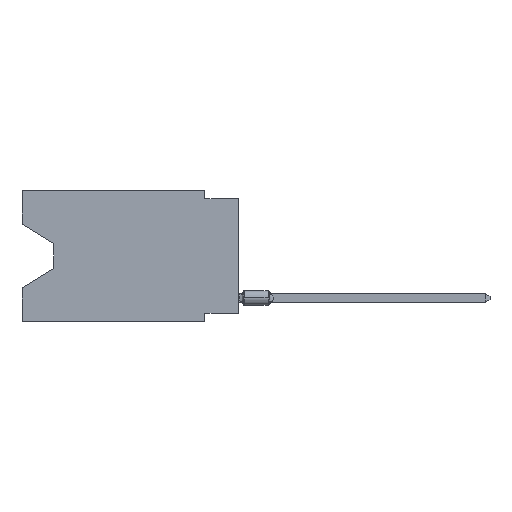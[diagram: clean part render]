
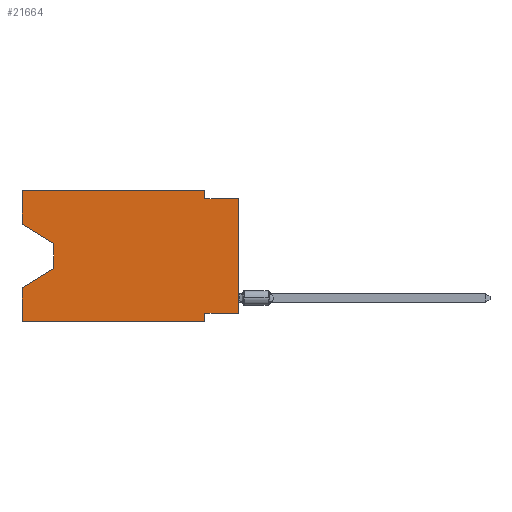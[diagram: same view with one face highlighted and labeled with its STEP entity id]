
A CAD part, left-side view. The second image highlights one B-rep face of the part: STEP entity #21664.
In plain terms, the highlighted planar face has unit normal (-1, 0, 0).
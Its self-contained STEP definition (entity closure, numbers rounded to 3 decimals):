
#264 = CARTESIAN_POINT ( 'NONE',  ( 0., 2.54, -0.635 ) ) ;
#439 = CARTESIAN_POINT ( 'NONE',  ( 0., 16.383, -2.546 ) ) ;
#1174 = VECTOR ( 'NONE', #18833, 1000. ) ;
#1178 = EDGE_CURVE ( 'NONE', #4654, #1676, #14690, .T. ) ;
#1676 = VERTEX_POINT ( 'NONE', #264 ) ;
#3243 = EDGE_CURVE ( 'NONE', #1676, #13821, #23773, .T. ) ;
#3281 = VECTOR ( 'NONE', #22348, 1000. ) ;
#4212 = VECTOR ( 'NONE', #21078, 1000. ) ;
#4266 = ORIENTED_EDGE ( 'NONE', *, *, #9920, .F. ) ;
#4325 = EDGE_CURVE ( 'NONE', #22542, #16185, #16788, .T. ) ;
#4528 = ORIENTED_EDGE ( 'NONE', *, *, #1178, .F. ) ;
#4582 = EDGE_CURVE ( 'NONE', #15624, #26573, #26738, .T. ) ;
#4654 = VERTEX_POINT ( 'NONE', #21216 ) ;
#4695 = DIRECTION ( 'NONE',  ( 0., -1., 0. ) ) ;
#4737 = EDGE_CURVE ( 'NONE', #22542, #13821, #25734, .T. ) ;
#5207 = EDGE_CURVE ( 'NONE', #12512, #17595, #5778, .T. ) ;
#5304 = DIRECTION ( 'NONE',  ( 0., 0., -1. ) ) ;
#5778 = LINE ( 'NONE', #7479, #24340 ) ;
#6340 = EDGE_CURVE ( 'NONE', #16185, #13503, #12993, .T. ) ;
#6423 = CARTESIAN_POINT ( 'NONE',  ( 0., 0., 0. ) ) ;
#6930 = VECTOR ( 'NONE', #19322, 1000. ) ;
#7479 = CARTESIAN_POINT ( 'NONE',  ( 0., 16.383, 0. ) ) ;
#7759 = CARTESIAN_POINT ( 'NONE',  ( 0., 16.383, 0. ) ) ;
#8341 = DIRECTION ( 'NONE',  ( 0., 0., -1. ) ) ;
#8631 = CARTESIAN_POINT ( 'NONE',  ( 0., 2.54, -9.906 ) ) ;
#8984 = VERTEX_POINT ( 'NONE', #7759 ) ;
#9226 = VECTOR ( 'NONE', #19690, 1000. ) ;
#9525 = CARTESIAN_POINT ( 'NONE',  ( 0., 16.383, -2.546 ) ) ;
#9920 = EDGE_CURVE ( 'NONE', #12831, #8984, #21634, .T. ) ;
#10760 = EDGE_CURVE ( 'NONE', #12831, #15624, #23974, .T. ) ;
#10925 = VECTOR ( 'NONE', #25218, 1000. ) ;
#10999 = CARTESIAN_POINT ( 'NONE',  ( 0., 2.54, -9.271 ) ) ;
#11297 = CARTESIAN_POINT ( 'NONE',  ( 0., 2.54, -9.906 ) ) ;
#11375 = CARTESIAN_POINT ( 'NONE',  ( 0., 0., -0.635 ) ) ;
#11657 = FACE_OUTER_BOUND ( 'NONE', #24232, .T. ) ;
#12475 = ORIENTED_EDGE ( 'NONE', *, *, #22771, .T. ) ;
#12502 = LINE ( 'NONE', #21076, #1174 ) ;
#12512 = VERTEX_POINT ( 'NONE', #18437 ) ;
#12831 = VERTEX_POINT ( 'NONE', #9525 ) ;
#12993 = LINE ( 'NONE', #8631, #6930 ) ;
#13197 = CARTESIAN_POINT ( 'NONE',  ( 0., 16.383, -7.36 ) ) ;
#13226 = LINE ( 'NONE', #15622, #9226 ) ;
#13503 = VERTEX_POINT ( 'NONE', #11297 ) ;
#13821 = VERTEX_POINT ( 'NONE', #19160 ) ;
#14046 = CARTESIAN_POINT ( 'NONE',  ( 0., 13.97, -4.013 ) ) ;
#14049 = DIRECTION ( 'NONE',  ( 1., 0., 0. ) ) ;
#14084 = AXIS2_PLACEMENT_3D ( 'NONE', #22908, #14049, #5304 ) ;
#14263 = ORIENTED_EDGE ( 'NONE', *, *, #10760, .T. ) ;
#14690 = LINE ( 'NONE', #19448, #17279 ) ;
#15227 = CARTESIAN_POINT ( 'NONE',  ( 0., 13.97, -5.893 ) ) ;
#15622 = CARTESIAN_POINT ( 'NONE',  ( 0., 16.383, -9.906 ) ) ;
#15624 = VERTEX_POINT ( 'NONE', #17982 ) ;
#15697 = CARTESIAN_POINT ( 'NONE',  ( 0., 16.383, 0. ) ) ;
#16185 = VERTEX_POINT ( 'NONE', #10999 ) ;
#16788 = LINE ( 'NONE', #21005, #23091 ) ;
#17279 = VECTOR ( 'NONE', #8341, 1000. ) ;
#17595 = VERTEX_POINT ( 'NONE', #13197 ) ;
#17880 = ORIENTED_EDGE ( 'NONE', *, *, #4325, .F. ) ;
#17982 = CARTESIAN_POINT ( 'NONE',  ( 0., 13.97, -4.013 ) ) ;
#18437 = CARTESIAN_POINT ( 'NONE',  ( 0., 16.383, -9.906 ) ) ;
#18833 = DIRECTION ( 'NONE',  ( 0., 0.855, -0.519 ) ) ;
#18965 = ORIENTED_EDGE ( 'NONE', *, *, #4582, .T. ) ;
#19160 = CARTESIAN_POINT ( 'NONE',  ( 0., 0., -0.635 ) ) ;
#19322 = DIRECTION ( 'NONE',  ( 0., 0., -1. ) ) ;
#19387 = ORIENTED_EDGE ( 'NONE', *, *, #4737, .T. ) ;
#19448 = CARTESIAN_POINT ( 'NONE',  ( 0., 2.54, 0. ) ) ;
#19564 = ORIENTED_EDGE ( 'NONE', *, *, #23654, .F. ) ;
#19690 = DIRECTION ( 'NONE',  ( 0., -1., 0. ) ) ;
#19952 = DIRECTION ( 'NONE',  ( 0., -1., 0. ) ) ;
#20038 = LINE ( 'NONE', #15697, #27733 ) ;
#20232 = PLANE ( 'NONE',  #14084 ) ;
#20842 = CARTESIAN_POINT ( 'NONE',  ( 0., 16.383, 0. ) ) ;
#20847 = DIRECTION ( 'NONE',  ( 0., 0., 1. ) ) ;
#20863 = DIRECTION ( 'NONE',  ( 0., 1., 0. ) ) ;
#21005 = CARTESIAN_POINT ( 'NONE',  ( 0., 0., -9.271 ) ) ;
#21076 = CARTESIAN_POINT ( 'NONE',  ( 0., 13.97, -5.893 ) ) ;
#21078 = DIRECTION ( 'NONE',  ( 0., 0., 1. ) ) ;
#21216 = CARTESIAN_POINT ( 'NONE',  ( 0., 2.54, 0. ) ) ;
#21634 = LINE ( 'NONE', #20842, #10925 ) ;
#21664 = ADVANCED_FACE ( 'NONE', ( #11657 ), #20232, .F. ) ;
#21850 = DIRECTION ( 'NONE',  ( 0., -0.855, -0.519 ) ) ;
#21916 = VECTOR ( 'NONE', #19952, 1000. ) ;
#22348 = DIRECTION ( 'NONE',  ( 0., 0., -1. ) ) ;
#22537 = VECTOR ( 'NONE', #21850, 1000. ) ;
#22542 = VERTEX_POINT ( 'NONE', #24268 ) ;
#22771 = EDGE_CURVE ( 'NONE', #12512, #13503, #13226, .T. ) ;
#22908 = CARTESIAN_POINT ( 'NONE',  ( 0., 16.383, 0. ) ) ;
#23091 = VECTOR ( 'NONE', #20863, 1000. ) ;
#23654 = EDGE_CURVE ( 'NONE', #8984, #4654, #20038, .T. ) ;
#23773 = LINE ( 'NONE', #11375, #21916 ) ;
#23974 = LINE ( 'NONE', #439, #22537 ) ;
#24054 = ORIENTED_EDGE ( 'NONE', *, *, #6340, .F. ) ;
#24232 = EDGE_LOOP ( 'NONE', ( #14263, #18965, #26900, #25641, #12475, #24054, #17880, #19387, #26878, #4528, #19564, #4266 ) ) ;
#24268 = CARTESIAN_POINT ( 'NONE',  ( 0., 0., -9.271 ) ) ;
#24340 = VECTOR ( 'NONE', #20847, 1000. ) ;
#24481 = EDGE_CURVE ( 'NONE', #26573, #17595, #12502, .T. ) ;
#25218 = DIRECTION ( 'NONE',  ( 0., 0., 1. ) ) ;
#25641 = ORIENTED_EDGE ( 'NONE', *, *, #5207, .F. ) ;
#25734 = LINE ( 'NONE', #6423, #4212 ) ;
#26573 = VERTEX_POINT ( 'NONE', #15227 ) ;
#26738 = LINE ( 'NONE', #14046, #3281 ) ;
#26878 = ORIENTED_EDGE ( 'NONE', *, *, #3243, .F. ) ;
#26900 = ORIENTED_EDGE ( 'NONE', *, *, #24481, .T. ) ;
#27733 = VECTOR ( 'NONE', #4695, 1000. ) ;
